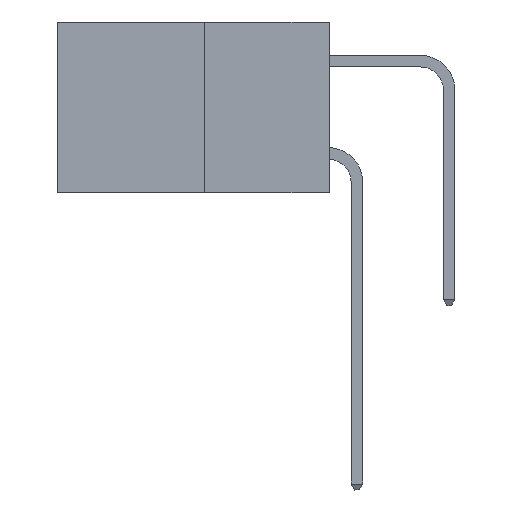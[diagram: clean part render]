
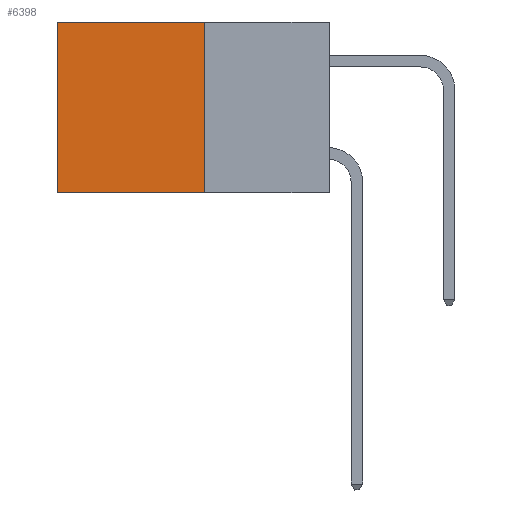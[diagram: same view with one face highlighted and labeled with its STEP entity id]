
A CAD part, left-side view. The second image highlights one B-rep face of the part: STEP entity #6398.
In plain terms, the highlighted planar face has unit normal (-1, 0, 0).
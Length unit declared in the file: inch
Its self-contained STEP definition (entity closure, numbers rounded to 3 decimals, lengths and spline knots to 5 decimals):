
#569 = AXIS2_PLACEMENT_3D ( 'NONE', #2029, #4099, #11075 ) ;
#606 = FACE_OUTER_BOUND ( 'NONE', #11096, .T. ) ;
#613 = DIRECTION ( 'NONE',  ( 0., 1., 0. ) ) ;
#798 = CARTESIAN_POINT ( 'NONE',  ( 0.277, 0.27, -0.37 ) ) ;
#1880 = ORIENTED_EDGE ( 'NONE', *, *, #11898, .F. ) ;
#1915 = CARTESIAN_POINT ( 'NONE',  ( 0.277, 0.27, 0. ) ) ;
#2029 = CARTESIAN_POINT ( 'NONE',  ( 0.277, 0.27, -0.37 ) ) ;
#2099 = VERTEX_POINT ( 'NONE', #1915 ) ;
#2478 = VERTEX_POINT ( 'NONE', #11474 ) ;
#2504 = CARTESIAN_POINT ( 'NONE',  ( 0.277, 0.27, 0. ) ) ;
#2542 = LINE ( 'NONE', #2504, #3145 ) ;
#2688 = ORIENTED_EDGE ( 'NONE', *, *, #3845, .T. ) ;
#3145 = VECTOR ( 'NONE', #9549, 39.37008 ) ;
#3683 = CARTESIAN_POINT ( 'NONE',  ( 0.277, 0.59, -0.37 ) ) ;
#3786 = ORIENTED_EDGE ( 'NONE', *, *, #10827, .F. ) ;
#3845 = EDGE_CURVE ( 'NONE', #2099, #2478, #2542, .T. ) ;
#4099 = DIRECTION ( 'NONE',  ( 1., 0., 0. ) ) ;
#4400 = LINE ( 'NONE', #10668, #6741 ) ;
#4529 = VERTEX_POINT ( 'NONE', #3683 ) ;
#4830 = VECTOR ( 'NONE', #613, 39.37008 ) ;
#5948 = CARTESIAN_POINT ( 'NONE',  ( 0.277, 0.59, -0.37 ) ) ;
#6040 = VECTOR ( 'NONE', #6970, 39.37008 ) ;
#6055 = PLANE ( 'NONE',  #569 ) ;
#6247 = VERTEX_POINT ( 'NONE', #798 ) ;
#6398 = ADVANCED_FACE ( 'NONE', ( #606 ), #6055, .F. ) ;
#6629 = CARTESIAN_POINT ( 'NONE',  ( 0.277, 0.27, -0.37 ) ) ;
#6741 = VECTOR ( 'NONE', #11652, 39.37008 ) ;
#6970 = DIRECTION ( 'NONE',  ( 0., 0., -1. ) ) ;
#7410 = ORIENTED_EDGE ( 'NONE', *, *, #8410, .T. ) ;
#8410 = EDGE_CURVE ( 'NONE', #2478, #4529, #8724, .T. ) ;
#8724 = LINE ( 'NONE', #5948, #6040 ) ;
#9549 = DIRECTION ( 'NONE',  ( 0., 1., 0. ) ) ;
#10143 = LINE ( 'NONE', #6629, #4830 ) ;
#10668 = CARTESIAN_POINT ( 'NONE',  ( 0.277, 0.27, -0.37 ) ) ;
#10827 = EDGE_CURVE ( 'NONE', #2099, #6247, #4400, .T. ) ;
#11075 = DIRECTION ( 'NONE',  ( 0., 0., -1. ) ) ;
#11096 = EDGE_LOOP ( 'NONE', ( #7410, #1880, #3786, #2688 ) ) ;
#11474 = CARTESIAN_POINT ( 'NONE',  ( 0.277, 0.59, 0. ) ) ;
#11652 = DIRECTION ( 'NONE',  ( 0., 0., -1. ) ) ;
#11898 = EDGE_CURVE ( 'NONE', #6247, #4529, #10143, .T. ) ;
